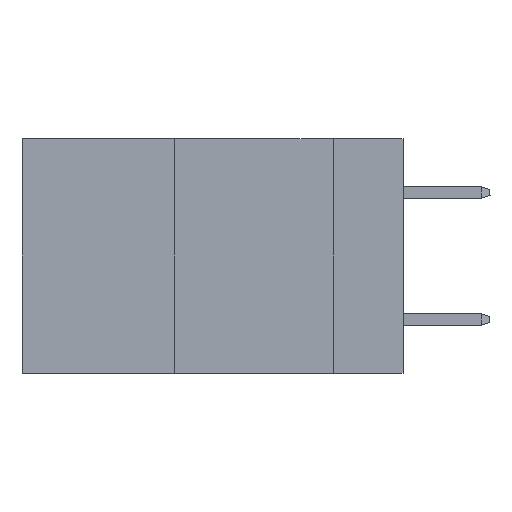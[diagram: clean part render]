
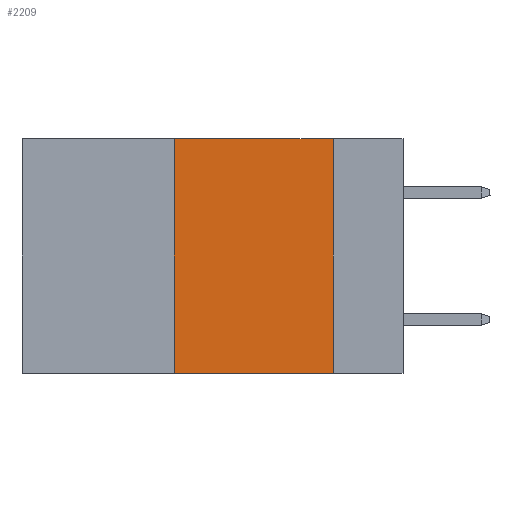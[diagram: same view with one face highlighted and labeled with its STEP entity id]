
A CAD part, left-side view. The second image highlights one B-rep face of the part: STEP entity #2209.
In plain terms, the highlighted planar face has unit normal (-1, 0, 0).
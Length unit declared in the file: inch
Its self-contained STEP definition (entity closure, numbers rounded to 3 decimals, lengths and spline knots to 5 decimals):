
#2009 = CARTESIAN_POINT ( 'NONE',  ( 0., 0.11, 0. ) ) ;
#2087 = EDGE_LOOP ( 'NONE', ( #29367, #21210, #40789, #35710 ) ) ;
#2209 = ADVANCED_FACE ( 'NONE', ( #13584 ), #27696, .F. ) ;
#2467 = LINE ( 'NONE', #2009, #18396 ) ;
#2858 = VECTOR ( 'NONE', #30827, 39.37008 ) ;
#4244 = EDGE_CURVE ( 'NONE', #32563, #21702, #24369, .T. ) ;
#8633 = DIRECTION ( 'NONE',  ( 0., -1., 0. ) ) ;
#13584 = FACE_OUTER_BOUND ( 'NONE', #2087, .T. ) ;
#14442 = VECTOR ( 'NONE', #8633, 39.37008 ) ;
#17305 = LINE ( 'NONE', #34369, #14442 ) ;
#17942 = VECTOR ( 'NONE', #31015, 39.37008 ) ;
#18396 = VECTOR ( 'NONE', #27171, 39.37008 ) ;
#20286 = CARTESIAN_POINT ( 'NONE',  ( 0., 0.6, 0. ) ) ;
#20797 = AXIS2_PLACEMENT_3D ( 'NONE', #20286, #41729, #33876 ) ;
#20853 = CARTESIAN_POINT ( 'NONE',  ( 0., 0.36, -0.37 ) ) ;
#21210 = ORIENTED_EDGE ( 'NONE', *, *, #4244, .F. ) ;
#21460 = CARTESIAN_POINT ( 'NONE',  ( 0., 0.11, 0. ) ) ;
#21702 = VERTEX_POINT ( 'NONE', #21460 ) ;
#23373 = CARTESIAN_POINT ( 'NONE',  ( 0., 0.36, 0. ) ) ;
#23677 = CARTESIAN_POINT ( 'NONE',  ( 0., 0.6, 0. ) ) ;
#24251 = VERTEX_POINT ( 'NONE', #30529 ) ;
#24369 = LINE ( 'NONE', #23677, #17942 ) ;
#25473 = EDGE_CURVE ( 'NONE', #21702, #24251, #2467, .T. ) ;
#27171 = DIRECTION ( 'NONE',  ( 0., 0., -1. ) ) ;
#27696 = PLANE ( 'NONE',  #20797 ) ;
#29367 = ORIENTED_EDGE ( 'NONE', *, *, #25473, .F. ) ;
#30529 = CARTESIAN_POINT ( 'NONE',  ( 0., 0.11, -0.37 ) ) ;
#30827 = DIRECTION ( 'NONE',  ( 0., 0., 1. ) ) ;
#31015 = DIRECTION ( 'NONE',  ( 0., -1., 0. ) ) ;
#32563 = VERTEX_POINT ( 'NONE', #23373 ) ;
#33876 = DIRECTION ( 'NONE',  ( 0., 0., -1. ) ) ;
#34064 = LINE ( 'NONE', #44683, #2858 ) ;
#34369 = CARTESIAN_POINT ( 'NONE',  ( 0., 0.6, -0.37 ) ) ;
#35710 = ORIENTED_EDGE ( 'NONE', *, *, #42261, .T. ) ;
#40789 = ORIENTED_EDGE ( 'NONE', *, *, #45311, .F. ) ;
#41729 = DIRECTION ( 'NONE',  ( 1., 0., 0. ) ) ;
#42261 = EDGE_CURVE ( 'NONE', #43669, #24251, #17305, .T. ) ;
#43669 = VERTEX_POINT ( 'NONE', #20853 ) ;
#44683 = CARTESIAN_POINT ( 'NONE',  ( 0., 0.36, 0. ) ) ;
#45311 = EDGE_CURVE ( 'NONE', #43669, #32563, #34064, .T. ) ;
